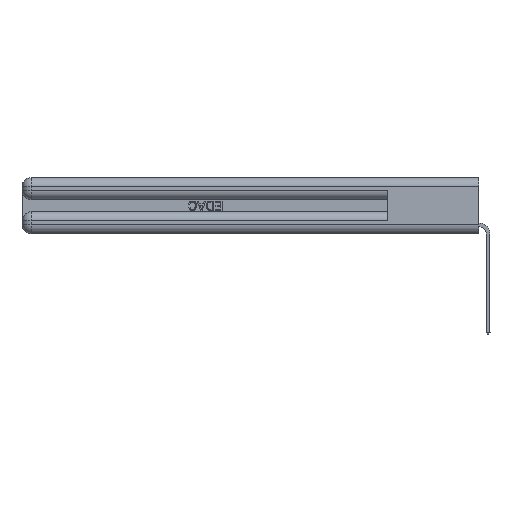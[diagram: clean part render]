
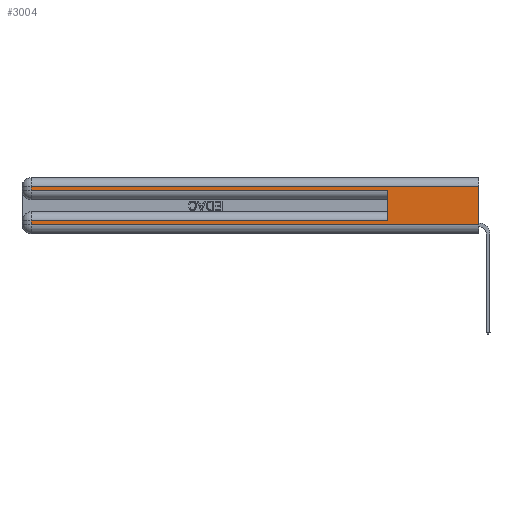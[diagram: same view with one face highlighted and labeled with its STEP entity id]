
A CAD part, left-side view. The second image highlights one B-rep face of the part: STEP entity #3004.
In plain terms, the highlighted planar face has unit normal (-1, 0, 0).
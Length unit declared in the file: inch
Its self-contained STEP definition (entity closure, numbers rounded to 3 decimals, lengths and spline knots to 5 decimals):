
#20 = CARTESIAN_POINT ( 'NONE',  ( 0., 2.94, 0.06 ) ) ;
#248 = VERTEX_POINT ( 'NONE', #15339 ) ;
#547 = DIRECTION ( 'NONE',  ( 0., 0., -1. ) ) ;
#1687 = DIRECTION ( 'NONE',  ( 0., 1., 0. ) ) ;
#1950 = ORIENTED_EDGE ( 'NONE', *, *, #17982, .T. ) ;
#2923 = DIRECTION ( 'NONE',  ( 0., 0., 1. ) ) ;
#3004 = ADVANCED_FACE ( 'NONE', ( #28056 ), #8064, .F. ) ;
#3421 = DIRECTION ( 'NONE',  ( 0., 0., -1. ) ) ;
#3623 = VERTEX_POINT ( 'NONE', #22822 ) ;
#3655 = LINE ( 'NONE', #9772, #25267 ) ;
#3667 = ORIENTED_EDGE ( 'NONE', *, *, #23956, .T. ) ;
#3959 = VECTOR ( 'NONE', #547, 39.37008 ) ;
#4006 = AXIS2_PLACEMENT_3D ( 'NONE', #16955, #15508, #20480 ) ;
#4188 = CARTESIAN_POINT ( 'NONE',  ( 0., 0., 0.31 ) ) ;
#4645 = LINE ( 'NONE', #25050, #13317 ) ;
#4689 = LINE ( 'NONE', #13520, #3959 ) ;
#5297 = VECTOR ( 'NONE', #1687, 39.37008 ) ;
#5539 = VECTOR ( 'NONE', #2923, 39.37008 ) ;
#5620 = LINE ( 'NONE', #7196, #28187 ) ;
#6210 = EDGE_CURVE ( 'NONE', #9062, #27216, #3655, .T. ) ;
#6986 = EDGE_CURVE ( 'NONE', #20740, #23042, #23366, .T. ) ;
#7196 = CARTESIAN_POINT ( 'NONE',  ( 0., 2.94, 0.37 ) ) ;
#8064 = PLANE ( 'NONE',  #4006 ) ;
#8624 = EDGE_LOOP ( 'NONE', ( #22436, #3667, #24970, #1950, #26532, #9896, #10741, #21925 ) ) ;
#9062 = VERTEX_POINT ( 'NONE', #26071 ) ;
#9144 = DIRECTION ( 'NONE',  ( 0., -1., 0. ) ) ;
#9211 = CARTESIAN_POINT ( 'NONE',  ( 0., 2.94, 0.285 ) ) ;
#9772 = CARTESIAN_POINT ( 'NONE',  ( 0., 2.94, 0.37 ) ) ;
#9896 = ORIENTED_EDGE ( 'NONE', *, *, #23345, .T. ) ;
#10741 = ORIENTED_EDGE ( 'NONE', *, *, #15943, .T. ) ;
#11397 = VERTEX_POINT ( 'NONE', #20 ) ;
#11652 = CARTESIAN_POINT ( 'NONE',  ( 0., 0.6, 0.085 ) ) ;
#13032 = LINE ( 'NONE', #17438, #15495 ) ;
#13317 = VECTOR ( 'NONE', #9144, 39.37008 ) ;
#13520 = CARTESIAN_POINT ( 'NONE',  ( 0., 0., 0.37 ) ) ;
#14310 = EDGE_CURVE ( 'NONE', #11397, #3623, #13032, .T. ) ;
#15339 = CARTESIAN_POINT ( 'NONE',  ( 0., 0., 0.31 ) ) ;
#15495 = VECTOR ( 'NONE', #21993, 39.37008 ) ;
#15508 = DIRECTION ( 'NONE',  ( 1., 0., 0. ) ) ;
#15943 = EDGE_CURVE ( 'NONE', #28210, #11397, #5620, .T. ) ;
#16140 = EDGE_CURVE ( 'NONE', #248, #3623, #4689, .T. ) ;
#16955 = CARTESIAN_POINT ( 'NONE',  ( 0., 0., 0.37 ) ) ;
#17062 = DIRECTION ( 'NONE',  ( 0., 0., -1. ) ) ;
#17438 = CARTESIAN_POINT ( 'NONE',  ( 0., 0., 0.06 ) ) ;
#17982 = EDGE_CURVE ( 'NONE', #27216, #23042, #4645, .T. ) ;
#19123 = CARTESIAN_POINT ( 'NONE',  ( 0., 2.94, 0.085 ) ) ;
#20449 = CARTESIAN_POINT ( 'NONE',  ( 0., 0., 0.085 ) ) ;
#20480 = DIRECTION ( 'NONE',  ( 0., 0., -1. ) ) ;
#20740 = VERTEX_POINT ( 'NONE', #11652 ) ;
#21925 = ORIENTED_EDGE ( 'NONE', *, *, #14310, .T. ) ;
#21993 = DIRECTION ( 'NONE',  ( 0., -1., 0. ) ) ;
#22323 = CARTESIAN_POINT ( 'NONE',  ( 0., 0.6, 0.285 ) ) ;
#22436 = ORIENTED_EDGE ( 'NONE', *, *, #16140, .F. ) ;
#22822 = CARTESIAN_POINT ( 'NONE',  ( 0., 0., 0.06 ) ) ;
#23042 = VERTEX_POINT ( 'NONE', #22323 ) ;
#23307 = VECTOR ( 'NONE', #27590, 39.37008 ) ;
#23345 = EDGE_CURVE ( 'NONE', #20740, #28210, #24976, .T. ) ;
#23366 = LINE ( 'NONE', #25256, #5539 ) ;
#23905 = LINE ( 'NONE', #4188, #5297 ) ;
#23956 = EDGE_CURVE ( 'NONE', #248, #9062, #23905, .T. ) ;
#24970 = ORIENTED_EDGE ( 'NONE', *, *, #6210, .T. ) ;
#24976 = LINE ( 'NONE', #20449, #23307 ) ;
#25050 = CARTESIAN_POINT ( 'NONE',  ( 0., 0., 0.285 ) ) ;
#25256 = CARTESIAN_POINT ( 'NONE',  ( 0., 0.6, 0.145 ) ) ;
#25267 = VECTOR ( 'NONE', #17062, 39.37008 ) ;
#26071 = CARTESIAN_POINT ( 'NONE',  ( 0., 2.94, 0.31 ) ) ;
#26532 = ORIENTED_EDGE ( 'NONE', *, *, #6986, .F. ) ;
#27216 = VERTEX_POINT ( 'NONE', #9211 ) ;
#27590 = DIRECTION ( 'NONE',  ( 0., 1., 0. ) ) ;
#28056 = FACE_OUTER_BOUND ( 'NONE', #8624, .T. ) ;
#28187 = VECTOR ( 'NONE', #3421, 39.37008 ) ;
#28210 = VERTEX_POINT ( 'NONE', #19123 ) ;
